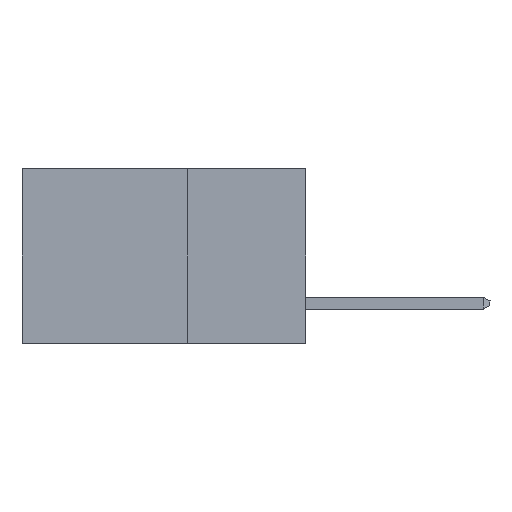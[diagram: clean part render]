
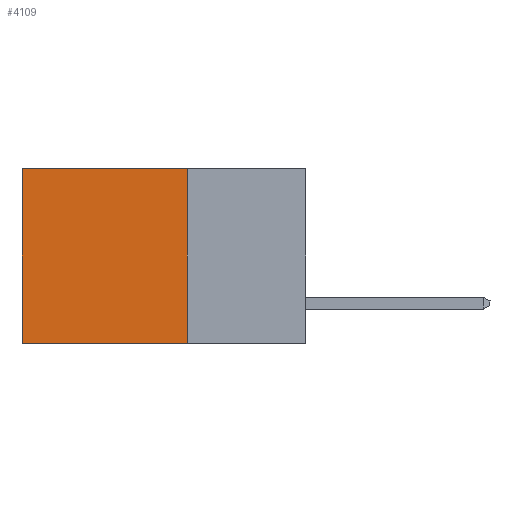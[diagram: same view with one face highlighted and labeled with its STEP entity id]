
A CAD part, left-side view. The second image highlights one B-rep face of the part: STEP entity #4109.
In plain terms, the highlighted planar face has unit normal (-1, 0, 0).
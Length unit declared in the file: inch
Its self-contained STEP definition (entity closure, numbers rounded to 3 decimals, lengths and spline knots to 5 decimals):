
#3 = LINE ( 'NONE', #4701, #7742 ) ;
#241 = ORIENTED_EDGE ( 'NONE', *, *, #3363, .F. ) ;
#502 = VERTEX_POINT ( 'NONE', #9143 ) ;
#785 = LINE ( 'NONE', #4366, #3107 ) ;
#1095 = EDGE_CURVE ( 'NONE', #7244, #3426, #2265, .T. ) ;
#1118 = DIRECTION ( 'NONE',  ( 0., 1., 0. ) ) ;
#1738 = DIRECTION ( 'NONE',  ( 0., 0., -1. ) ) ;
#2174 = DIRECTION ( 'NONE',  ( 0., 0., -1. ) ) ;
#2265 = LINE ( 'NONE', #7276, #4503 ) ;
#2413 = FACE_OUTER_BOUND ( 'NONE', #7802, .T. ) ;
#2467 = CARTESIAN_POINT ( 'NONE',  ( 0.298, 0.6, 0. ) ) ;
#3107 = VECTOR ( 'NONE', #1118, 39.37008 ) ;
#3363 = EDGE_CURVE ( 'NONE', #9637, #502, #3, .T. ) ;
#3426 = VERTEX_POINT ( 'NONE', #6586 ) ;
#4065 = ORIENTED_EDGE ( 'NONE', *, *, #1095, .T. ) ;
#4109 = ADVANCED_FACE ( 'NONE', ( #2413 ), #8085, .F. ) ;
#4366 = CARTESIAN_POINT ( 'NONE',  ( 0.298, 0.25, -0.37 ) ) ;
#4488 = ORIENTED_EDGE ( 'NONE', *, *, #4528, .F. ) ;
#4503 = VECTOR ( 'NONE', #2174, 39.37008 ) ;
#4528 = EDGE_CURVE ( 'NONE', #502, #3426, #785, .T. ) ;
#4564 = ORIENTED_EDGE ( 'NONE', *, *, #6251, .T. ) ;
#4701 = CARTESIAN_POINT ( 'NONE',  ( 0.298, 0.25, 0. ) ) ;
#5307 = DIRECTION ( 'NONE',  ( 1., 0., 0. ) ) ;
#5995 = VECTOR ( 'NONE', #7453, 39.37008 ) ;
#6251 = EDGE_CURVE ( 'NONE', #9637, #7244, #7517, .T. ) ;
#6586 = CARTESIAN_POINT ( 'NONE',  ( 0.298, 0.6, -0.37 ) ) ;
#6629 = CARTESIAN_POINT ( 'NONE',  ( 0.298, 0.25, 0. ) ) ;
#6788 = CARTESIAN_POINT ( 'NONE',  ( 0.298, 0.25, 0. ) ) ;
#7244 = VERTEX_POINT ( 'NONE', #2467 ) ;
#7276 = CARTESIAN_POINT ( 'NONE',  ( 0.298, 0.6, 0. ) ) ;
#7346 = CARTESIAN_POINT ( 'NONE',  ( 0.298, 0.25, 0. ) ) ;
#7453 = DIRECTION ( 'NONE',  ( 0., 1., 0. ) ) ;
#7517 = LINE ( 'NONE', #6629, #5995 ) ;
#7573 = AXIS2_PLACEMENT_3D ( 'NONE', #7346, #5307, #9197 ) ;
#7742 = VECTOR ( 'NONE', #1738, 39.37008 ) ;
#7802 = EDGE_LOOP ( 'NONE', ( #4065, #4488, #241, #4564 ) ) ;
#8085 = PLANE ( 'NONE',  #7573 ) ;
#9143 = CARTESIAN_POINT ( 'NONE',  ( 0.298, 0.25, -0.37 ) ) ;
#9197 = DIRECTION ( 'NONE',  ( 0., 0., -1. ) ) ;
#9637 = VERTEX_POINT ( 'NONE', #6788 ) ;
